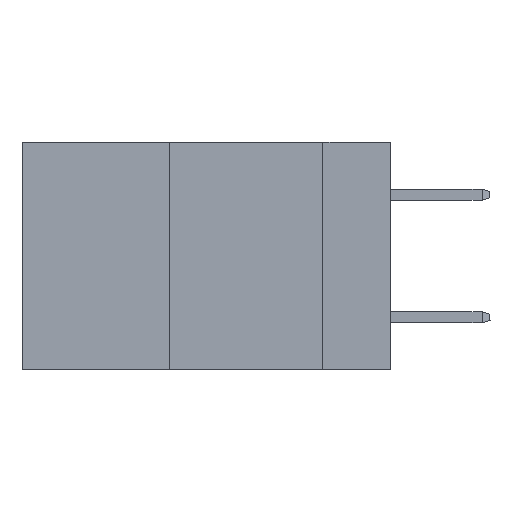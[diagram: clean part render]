
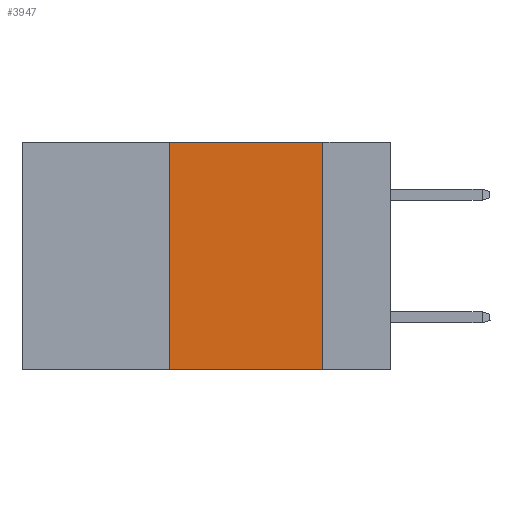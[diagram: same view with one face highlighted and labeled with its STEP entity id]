
A CAD part, left-side view. The second image highlights one B-rep face of the part: STEP entity #3947.
In plain terms, the highlighted planar face has unit normal (-1, 0, 0).
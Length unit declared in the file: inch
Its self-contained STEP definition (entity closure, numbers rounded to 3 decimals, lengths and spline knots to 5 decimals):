
#34 = CARTESIAN_POINT ( 'NONE',  ( 0., 0.11, 0. ) ) ;
#656 = VERTEX_POINT ( 'NONE', #10227 ) ;
#687 = EDGE_CURVE ( 'NONE', #7813, #20938, #17878, .T. ) ;
#894 = CARTESIAN_POINT ( 'NONE',  ( 0., 0.6, 0. ) ) ;
#1687 = VERTEX_POINT ( 'NONE', #34 ) ;
#1770 = ORIENTED_EDGE ( 'NONE', *, *, #8859, .F. ) ;
#2165 = ORIENTED_EDGE ( 'NONE', *, *, #19267, .F. ) ;
#2692 = ORIENTED_EDGE ( 'NONE', *, *, #687, .T. ) ;
#2799 = DIRECTION ( 'NONE',  ( 0., 0., -1. ) ) ;
#3721 = ORIENTED_EDGE ( 'NONE', *, *, #15749, .F. ) ;
#3947 = ADVANCED_FACE ( 'NONE', ( #16394 ), #11855, .F. ) ;
#4749 = VECTOR ( 'NONE', #20758, 39.37008 ) ;
#4972 = DIRECTION ( 'NONE',  ( 0., 0., -1. ) ) ;
#6826 = VECTOR ( 'NONE', #15789, 39.37008 ) ;
#6871 = CARTESIAN_POINT ( 'NONE',  ( 0., 0.6, 0. ) ) ;
#7813 = VERTEX_POINT ( 'NONE', #19894 ) ;
#7861 = VECTOR ( 'NONE', #15588, 39.37008 ) ;
#8577 = CARTESIAN_POINT ( 'NONE',  ( 0., 0.11, 0. ) ) ;
#8859 = EDGE_CURVE ( 'NONE', #656, #1687, #16320, .T. ) ;
#10227 = CARTESIAN_POINT ( 'NONE',  ( 0., 0.36, 0. ) ) ;
#11132 = VECTOR ( 'NONE', #4972, 39.37008 ) ;
#11855 = PLANE ( 'NONE',  #21431 ) ;
#12607 = EDGE_LOOP ( 'NONE', ( #3721, #1770, #2165, #2692 ) ) ;
#13638 = DIRECTION ( 'NONE',  ( 1., 0., 0. ) ) ;
#13690 = CARTESIAN_POINT ( 'NONE',  ( 0., 0.36, 0. ) ) ;
#14855 = LINE ( 'NONE', #13690, #4749 ) ;
#15588 = DIRECTION ( 'NONE',  ( 0., -1., 0. ) ) ;
#15749 = EDGE_CURVE ( 'NONE', #1687, #20938, #20506, .T. ) ;
#15789 = DIRECTION ( 'NONE',  ( 0., -1., 0. ) ) ;
#16320 = LINE ( 'NONE', #6871, #6826 ) ;
#16394 = FACE_OUTER_BOUND ( 'NONE', #12607, .T. ) ;
#17878 = LINE ( 'NONE', #19099, #7861 ) ;
#18943 = CARTESIAN_POINT ( 'NONE',  ( 0., 0.11, -0.37 ) ) ;
#19099 = CARTESIAN_POINT ( 'NONE',  ( 0., 0.6, -0.37 ) ) ;
#19267 = EDGE_CURVE ( 'NONE', #7813, #656, #14855, .T. ) ;
#19894 = CARTESIAN_POINT ( 'NONE',  ( 0., 0.36, -0.37 ) ) ;
#20506 = LINE ( 'NONE', #8577, #11132 ) ;
#20758 = DIRECTION ( 'NONE',  ( 0., 0., 1. ) ) ;
#20938 = VERTEX_POINT ( 'NONE', #18943 ) ;
#21431 = AXIS2_PLACEMENT_3D ( 'NONE', #894, #13638, #2799 ) ;
